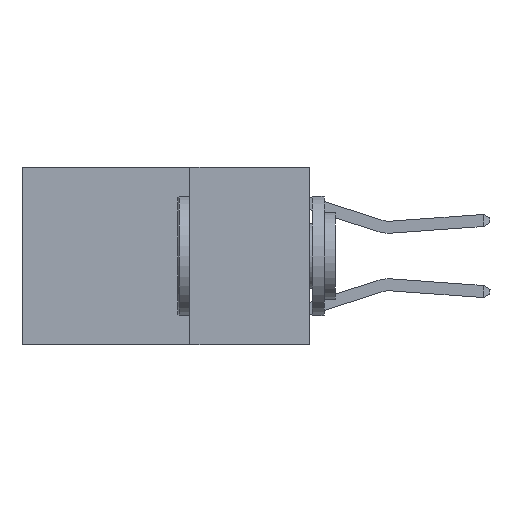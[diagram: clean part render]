
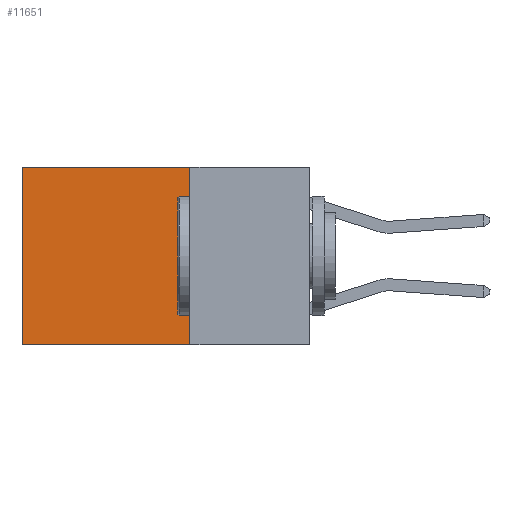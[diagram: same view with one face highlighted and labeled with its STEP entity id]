
A CAD part, left-side view. The second image highlights one B-rep face of the part: STEP entity #11651.
In plain terms, the highlighted planar face has unit normal (-1, 0, 0).
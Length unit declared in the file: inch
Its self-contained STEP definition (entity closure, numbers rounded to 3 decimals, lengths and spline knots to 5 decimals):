
#44 = CARTESIAN_POINT ( 'NONE',  ( 0.2625, 0.6, 0. ) ) ;
#140 = LINE ( 'NONE', #3696, #14089 ) ;
#317 = CARTESIAN_POINT ( 'NONE',  ( 0.2625, 0.25, 0. ) ) ;
#1721 = DIRECTION ( 'NONE',  ( 1., 0., 0. ) ) ;
#2367 = CARTESIAN_POINT ( 'NONE',  ( 0.2625, 0.6, -0.37 ) ) ;
#2651 = EDGE_CURVE ( 'NONE', #8801, #5015, #10056, .T. ) ;
#2934 = VECTOR ( 'NONE', #5133, 39.37008 ) ;
#3009 = EDGE_CURVE ( 'NONE', #14928, #3438, #5331, .T. ) ;
#3340 = ORIENTED_EDGE ( 'NONE', *, *, #12431, .F. ) ;
#3432 = DIRECTION ( 'NONE',  ( 0., 0., -1. ) ) ;
#3438 = VERTEX_POINT ( 'NONE', #2367 ) ;
#3696 = CARTESIAN_POINT ( 'NONE',  ( 0.2625, 0.25, 0. ) ) ;
#4110 = DIRECTION ( 'NONE',  ( 0., 0., -1. ) ) ;
#5015 = VERTEX_POINT ( 'NONE', #5648 ) ;
#5133 = DIRECTION ( 'NONE',  ( 0., 0., -1. ) ) ;
#5331 = LINE ( 'NONE', #14338, #2934 ) ;
#5648 = CARTESIAN_POINT ( 'NONE',  ( 0.2625, 0.25, -0.37 ) ) ;
#6478 = ORIENTED_EDGE ( 'NONE', *, *, #2651, .F. ) ;
#7101 = AXIS2_PLACEMENT_3D ( 'NONE', #11918, #1721, #4110 ) ;
#7494 = VECTOR ( 'NONE', #3432, 39.37008 ) ;
#7691 = FACE_OUTER_BOUND ( 'NONE', #11753, .T. ) ;
#7854 = VECTOR ( 'NONE', #13899, 39.37008 ) ;
#8801 = VERTEX_POINT ( 'NONE', #317 ) ;
#8849 = ORIENTED_EDGE ( 'NONE', *, *, #10019, .T. ) ;
#9340 = DIRECTION ( 'NONE',  ( 0., 1., 0. ) ) ;
#10019 = EDGE_CURVE ( 'NONE', #8801, #14928, #140, .T. ) ;
#10056 = LINE ( 'NONE', #12459, #7494 ) ;
#10137 = CARTESIAN_POINT ( 'NONE',  ( 0.2625, 0.25, -0.37 ) ) ;
#11651 = ADVANCED_FACE ( 'NONE', ( #7691 ), #15185, .F. ) ;
#11753 = EDGE_LOOP ( 'NONE', ( #15093, #3340, #6478, #8849 ) ) ;
#11918 = CARTESIAN_POINT ( 'NONE',  ( 0.2625, 0.25, 0. ) ) ;
#12431 = EDGE_CURVE ( 'NONE', #5015, #3438, #14502, .T. ) ;
#12459 = CARTESIAN_POINT ( 'NONE',  ( 0.2625, 0.25, 0. ) ) ;
#13899 = DIRECTION ( 'NONE',  ( 0., 1., 0. ) ) ;
#14089 = VECTOR ( 'NONE', #9340, 39.37008 ) ;
#14338 = CARTESIAN_POINT ( 'NONE',  ( 0.2625, 0.6, 0. ) ) ;
#14502 = LINE ( 'NONE', #10137, #7854 ) ;
#14928 = VERTEX_POINT ( 'NONE', #44 ) ;
#15093 = ORIENTED_EDGE ( 'NONE', *, *, #3009, .T. ) ;
#15185 = PLANE ( 'NONE',  #7101 ) ;
